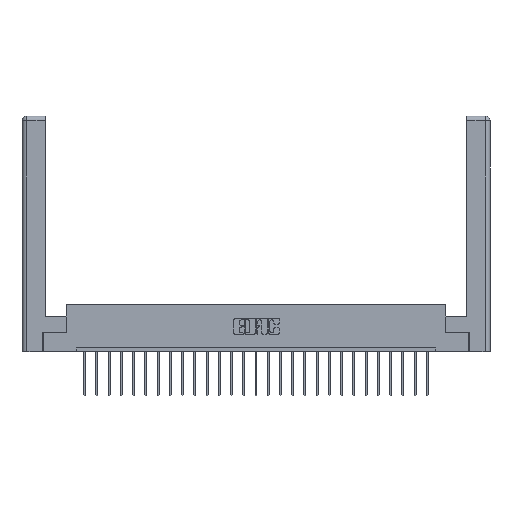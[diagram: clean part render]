
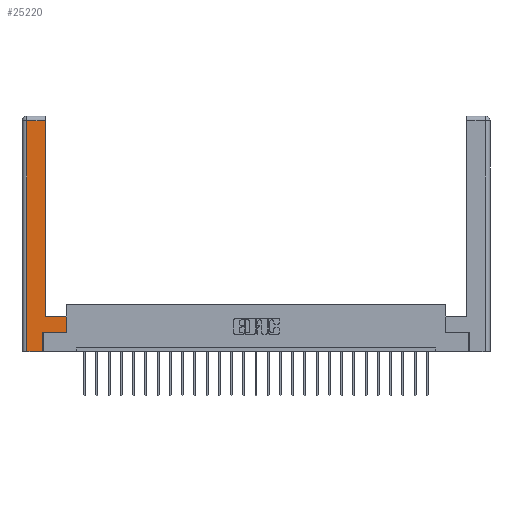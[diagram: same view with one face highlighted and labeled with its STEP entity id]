
A CAD part, top view. The second image highlights one B-rep face of the part: STEP entity #25220.
In plain terms, the highlighted planar face has unit normal (0, 0, 1).
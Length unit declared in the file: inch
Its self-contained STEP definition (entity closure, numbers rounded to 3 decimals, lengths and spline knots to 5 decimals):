
#429 = DIRECTION ( 'NONE',  ( 0., 1., 0. ) ) ;
#559 = ORIENTED_EDGE ( 'NONE', *, *, #1177, .T. ) ;
#731 = LINE ( 'NONE', #4449, #5089 ) ;
#1177 = EDGE_CURVE ( 'NONE', #25724, #23555, #21990, .T. ) ;
#1231 = VECTOR ( 'NONE', #5190, 39.37008 ) ;
#1343 = VERTEX_POINT ( 'NONE', #9260 ) ;
#1483 = EDGE_CURVE ( 'NONE', #18978, #1343, #731, .T. ) ;
#3443 = CARTESIAN_POINT ( 'NONE',  ( 0., 0., 0. ) ) ;
#3810 = CARTESIAN_POINT ( 'NONE',  ( 0.295, 0.45, 0. ) ) ;
#4153 = CARTESIAN_POINT ( 'NONE',  ( 0.0615, 2.94, 0. ) ) ;
#4449 = CARTESIAN_POINT ( 'NONE',  ( 0.565, 0.245, 0. ) ) ;
#5089 = VECTOR ( 'NONE', #22291, 39.37008 ) ;
#5190 = DIRECTION ( 'NONE',  ( -1., 0., 0. ) ) ;
#5714 = PLANE ( 'NONE',  #24498 ) ;
#6037 = VECTOR ( 'NONE', #22176, 39.37008 ) ;
#6290 = ORIENTED_EDGE ( 'NONE', *, *, #10233, .T. ) ;
#6302 = DIRECTION ( 'NONE',  ( 0., -1., 0. ) ) ;
#6349 = CARTESIAN_POINT ( 'NONE',  ( 0.265, 0., 0. ) ) ;
#6545 = LINE ( 'NONE', #17185, #1231 ) ;
#6584 = EDGE_CURVE ( 'NONE', #11663, #16610, #23619, .T. ) ;
#7149 = DIRECTION ( 'NONE',  ( 0., 1., 0. ) ) ;
#7289 = FACE_OUTER_BOUND ( 'NONE', #12334, .T. ) ;
#8933 = VECTOR ( 'NONE', #20801, 39.37008 ) ;
#9204 = VERTEX_POINT ( 'NONE', #18158 ) ;
#9260 = CARTESIAN_POINT ( 'NONE',  ( 0.565, 0.245, 0. ) ) ;
#9509 = DIRECTION ( 'NONE',  ( 0., 0., -1. ) ) ;
#9846 = CARTESIAN_POINT ( 'NONE',  ( 0.265, 0.245, 0. ) ) ;
#10233 = EDGE_CURVE ( 'NONE', #12667, #25724, #24860, .T. ) ;
#11205 = CARTESIAN_POINT ( 'NONE',  ( 0.0615, 0., 0. ) ) ;
#11663 = VERTEX_POINT ( 'NONE', #3810 ) ;
#12334 = EDGE_LOOP ( 'NONE', ( #22869, #25253, #6290, #559, #13460, #16656, #25174, #19259 ) ) ;
#12667 = VERTEX_POINT ( 'NONE', #12923 ) ;
#12923 = CARTESIAN_POINT ( 'NONE',  ( 0.0615, 2.94, 0. ) ) ;
#13460 = ORIENTED_EDGE ( 'NONE', *, *, #22238, .T. ) ;
#14638 = CARTESIAN_POINT ( 'NONE',  ( 0.265, 0., 0. ) ) ;
#15250 = VECTOR ( 'NONE', #7149, 39.37008 ) ;
#15561 = VECTOR ( 'NONE', #15822, 39.37008 ) ;
#15822 = DIRECTION ( 'NONE',  ( -1., 0., 0. ) ) ;
#16383 = CARTESIAN_POINT ( 'NONE',  ( 0.0615, 0., 0. ) ) ;
#16610 = VERTEX_POINT ( 'NONE', #22264 ) ;
#16656 = ORIENTED_EDGE ( 'NONE', *, *, #1483, .T. ) ;
#17185 = CARTESIAN_POINT ( 'NONE',  ( 0.295, 0.45, 0. ) ) ;
#17662 = VECTOR ( 'NONE', #429, 39.37008 ) ;
#18158 = CARTESIAN_POINT ( 'NONE',  ( 0.565, 0.45, 0. ) ) ;
#18349 = CARTESIAN_POINT ( 'NONE',  ( 0.565, 0.45, 0. ) ) ;
#18978 = VERTEX_POINT ( 'NONE', #9846 ) ;
#19133 = CARTESIAN_POINT ( 'NONE',  ( 0.265, 0.245, 0. ) ) ;
#19259 = ORIENTED_EDGE ( 'NONE', *, *, #21139, .T. ) ;
#20108 = EDGE_CURVE ( 'NONE', #1343, #9204, #21074, .T. ) ;
#20717 = CARTESIAN_POINT ( 'NONE',  ( 0.295, 3., 0. ) ) ;
#20801 = DIRECTION ( 'NONE',  ( 0., 1., 0. ) ) ;
#21074 = LINE ( 'NONE', #18349, #17662 ) ;
#21139 = EDGE_CURVE ( 'NONE', #9204, #11663, #6545, .T. ) ;
#21990 = LINE ( 'NONE', #6349, #6037 ) ;
#22176 = DIRECTION ( 'NONE',  ( 1., 0., 0. ) ) ;
#22238 = EDGE_CURVE ( 'NONE', #23555, #18978, #23971, .T. ) ;
#22264 = CARTESIAN_POINT ( 'NONE',  ( 0.295, 2.94, 0. ) ) ;
#22291 = DIRECTION ( 'NONE',  ( 1., 0., 0. ) ) ;
#22378 = LINE ( 'NONE', #4153, #15561 ) ;
#22869 = ORIENTED_EDGE ( 'NONE', *, *, #6584, .T. ) ;
#22933 = EDGE_CURVE ( 'NONE', #16610, #12667, #22378, .T. ) ;
#23481 = DIRECTION ( 'NONE',  ( -1., 0., 0. ) ) ;
#23555 = VERTEX_POINT ( 'NONE', #14638 ) ;
#23619 = LINE ( 'NONE', #20717, #8933 ) ;
#23641 = VECTOR ( 'NONE', #6302, 39.37008 ) ;
#23971 = LINE ( 'NONE', #19133, #15250 ) ;
#24498 = AXIS2_PLACEMENT_3D ( 'NONE', #3443, #9509, #23481 ) ;
#24860 = LINE ( 'NONE', #16383, #23641 ) ;
#25174 = ORIENTED_EDGE ( 'NONE', *, *, #20108, .T. ) ;
#25220 = ADVANCED_FACE ( 'NONE', ( #7289 ), #5714, .F. ) ;
#25253 = ORIENTED_EDGE ( 'NONE', *, *, #22933, .T. ) ;
#25724 = VERTEX_POINT ( 'NONE', #11205 ) ;
